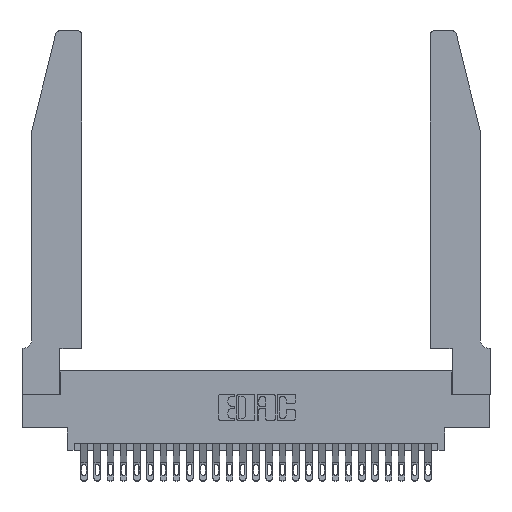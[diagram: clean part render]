
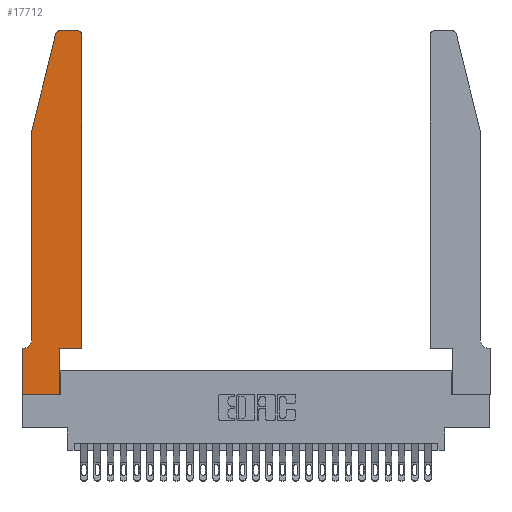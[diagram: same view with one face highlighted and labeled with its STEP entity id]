
A CAD part, top view. The second image highlights one B-rep face of the part: STEP entity #17712.
In plain terms, the highlighted planar face has unit normal (0, 0, 1).
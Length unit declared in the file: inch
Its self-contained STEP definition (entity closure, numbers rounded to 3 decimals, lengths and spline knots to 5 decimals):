
#638 = DIRECTION ( 'NONE',  ( 1., 0., 0. ) ) ;
#938 = VERTEX_POINT ( 'NONE', #22571 ) ;
#1286 = VERTEX_POINT ( 'NONE', #9032 ) ;
#1405 = AXIS2_PLACEMENT_3D ( 'NONE', #23999, #10902, #26207 ) ;
#1491 = CARTESIAN_POINT ( 'NONE',  ( 0.2865, 0.35, 0.37 ) ) ;
#2032 = DIRECTION ( 'NONE',  ( 1., 0., 0. ) ) ;
#2390 = CARTESIAN_POINT ( 'NONE',  ( 0., 0., 0.37 ) ) ;
#2399 = VERTEX_POINT ( 'NONE', #20181 ) ;
#2743 = ORIENTED_EDGE ( 'NONE', *, *, #19692, .T. ) ;
#2772 = VERTEX_POINT ( 'NONE', #26494 ) ;
#2855 = CARTESIAN_POINT ( 'NONE',  ( 0.4505, 0.35, 0.37 ) ) ;
#3191 = VECTOR ( 'NONE', #9762, 39.37008 ) ;
#3210 = ORIENTED_EDGE ( 'NONE', *, *, #19323, .T. ) ;
#3526 = LINE ( 'NONE', #24696, #26150 ) ;
#4059 = ORIENTED_EDGE ( 'NONE', *, *, #17505, .T. ) ;
#4582 = CARTESIAN_POINT ( 'NONE',  ( 0.0755, 2., 0.37 ) ) ;
#4821 = LINE ( 'NONE', #14977, #21586 ) ;
#5049 = ORIENTED_EDGE ( 'NONE', *, *, #12039, .T. ) ;
#5088 = DIRECTION ( 'NONE',  ( 0., 1., 0. ) ) ;
#5116 = ORIENTED_EDGE ( 'NONE', *, *, #13300, .T. ) ;
#5153 = AXIS2_PLACEMENT_3D ( 'NONE', #17276, #15197, #2032 ) ;
#6018 = VECTOR ( 'NONE', #24577, 39.37008 ) ;
#6329 = EDGE_CURVE ( 'NONE', #21389, #938, #27459, .T. ) ;
#6726 = DIRECTION ( 'NONE',  ( -1., 0., 0. ) ) ;
#6856 = DIRECTION ( 'NONE',  ( 0., -1., 0. ) ) ;
#6885 = DIRECTION ( 'NONE',  ( 0., 0., -1. ) ) ;
#6930 = LINE ( 'NONE', #2390, #23001 ) ;
#7084 = CARTESIAN_POINT ( 'NONE',  ( 0.4505, 0.35, 0.37 ) ) ;
#7373 = CARTESIAN_POINT ( 'NONE',  ( 0.4205, 2.75, 0.37 ) ) ;
#7693 = VECTOR ( 'NONE', #6726, 39.37008 ) ;
#8584 = CIRCLE ( 'NONE', #25892, 0.07 ) ;
#9032 = CARTESIAN_POINT ( 'NONE',  ( 0.0055, 0.35, 0.37 ) ) ;
#9314 = VECTOR ( 'NONE', #5088, 39.37008 ) ;
#9665 = ORIENTED_EDGE ( 'NONE', *, *, #13156, .T. ) ;
#9762 = DIRECTION ( 'NONE',  ( 1., 0., 0. ) ) ;
#10742 = FACE_OUTER_BOUND ( 'NONE', #16281, .T. ) ;
#10902 = DIRECTION ( 'NONE',  ( 0., 0., 1. ) ) ;
#11002 = VECTOR ( 'NONE', #25261, 39.37008 ) ;
#11259 = ORIENTED_EDGE ( 'NONE', *, *, #19066, .T. ) ;
#11550 = VERTEX_POINT ( 'NONE', #18581 ) ;
#11599 = ORIENTED_EDGE ( 'NONE', *, *, #16405, .T. ) ;
#11856 = LINE ( 'NONE', #7084, #6018 ) ;
#12039 = EDGE_CURVE ( 'NONE', #28290, #21389, #11856, .T. ) ;
#12504 = AXIS2_PLACEMENT_3D ( 'NONE', #26952, #13868, #638 ) ;
#13156 = EDGE_CURVE ( 'NONE', #16662, #2772, #19318, .T. ) ;
#13300 = EDGE_CURVE ( 'NONE', #11550, #22076, #3526, .T. ) ;
#13771 = LINE ( 'NONE', #23049, #11002 ) ;
#13868 = DIRECTION ( 'NONE',  ( 0., 0., 1. ) ) ;
#14195 = CIRCLE ( 'NONE', #12504, 0.03 ) ;
#14228 = LINE ( 'NONE', #18942, #3191 ) ;
#14344 = ORIENTED_EDGE ( 'NONE', *, *, #18013, .T. ) ;
#14977 = CARTESIAN_POINT ( 'NONE',  ( 0.0755, 0.35, 0.37 ) ) ;
#15197 = DIRECTION ( 'NONE',  ( 0., 0., 1. ) ) ;
#15374 = EDGE_CURVE ( 'NONE', #19605, #24996, #6930, .T. ) ;
#15944 = CARTESIAN_POINT ( 'NONE',  ( 0.0755, 0.42, 0.37 ) ) ;
#16281 = EDGE_LOOP ( 'NONE', ( #9665, #14344, #5116, #11259, #2743, #23636, #17816, #4059, #3210, #5049, #23106, #11599 ) ) ;
#16405 = EDGE_CURVE ( 'NONE', #938, #16662, #24469, .T. ) ;
#16662 = VERTEX_POINT ( 'NONE', #7373 ) ;
#17276 = CARTESIAN_POINT ( 'NONE',  ( 0., 0.35, 0.37 ) ) ;
#17376 = CARTESIAN_POINT ( 'NONE',  ( 0., 0.35, 0.37 ) ) ;
#17505 = EDGE_CURVE ( 'NONE', #24996, #2399, #14228, .T. ) ;
#17712 = ADVANCED_FACE ( 'NONE', ( #10742 ), #28287, .T. ) ;
#17816 = ORIENTED_EDGE ( 'NONE', *, *, #15374, .T. ) ;
#17996 = VERTEX_POINT ( 'NONE', #15944 ) ;
#18013 = EDGE_CURVE ( 'NONE', #2772, #11550, #14195, .T. ) ;
#18558 = VECTOR ( 'NONE', #22092, 39.37008 ) ;
#18581 = CARTESIAN_POINT ( 'NONE',  ( 0.25487, 2.72718, 0.37 ) ) ;
#18942 = CARTESIAN_POINT ( 'NONE',  ( 0., 0., 0.37 ) ) ;
#19066 = EDGE_CURVE ( 'NONE', #22076, #17996, #24360, .T. ) ;
#19318 = LINE ( 'NONE', #21998, #7693 ) ;
#19323 = EDGE_CURVE ( 'NONE', #2399, #28290, #13771, .T. ) ;
#19605 = VERTEX_POINT ( 'NONE', #17376 ) ;
#19692 = EDGE_CURVE ( 'NONE', #17996, #1286, #8584, .T. ) ;
#19978 = CARTESIAN_POINT ( 'NONE',  ( 0.0055, 0.42, 0.37 ) ) ;
#20181 = CARTESIAN_POINT ( 'NONE',  ( 0.2865, 0., 0.37 ) ) ;
#21389 = VERTEX_POINT ( 'NONE', #27549 ) ;
#21586 = VECTOR ( 'NONE', #23666, 39.37008 ) ;
#21998 = CARTESIAN_POINT ( 'NONE',  ( 0.2605, 2.75, 0.37 ) ) ;
#22076 = VERTEX_POINT ( 'NONE', #27878 ) ;
#22092 = DIRECTION ( 'NONE',  ( 0., -1., 0. ) ) ;
#22157 = DIRECTION ( 'NONE',  ( -1., 0., 0. ) ) ;
#22571 = CARTESIAN_POINT ( 'NONE',  ( 0.4505, 2.72, 0.37 ) ) ;
#23001 = VECTOR ( 'NONE', #6856, 39.37008 ) ;
#23049 = CARTESIAN_POINT ( 'NONE',  ( 0.2865, 0.35, 0.37 ) ) ;
#23106 = ORIENTED_EDGE ( 'NONE', *, *, #6329, .T. ) ;
#23636 = ORIENTED_EDGE ( 'NONE', *, *, #23710, .T. ) ;
#23666 = DIRECTION ( 'NONE',  ( -1., 0., 0. ) ) ;
#23710 = EDGE_CURVE ( 'NONE', #1286, #19605, #4821, .T. ) ;
#23999 = CARTESIAN_POINT ( 'NONE',  ( 0.4205, 2.72, 0.37 ) ) ;
#24360 = LINE ( 'NONE', #4582, #18558 ) ;
#24469 = CIRCLE ( 'NONE', #1405, 0.03 ) ;
#24577 = DIRECTION ( 'NONE',  ( 1., 0., 0. ) ) ;
#24606 = DIRECTION ( 'NONE',  ( -0.239, -0.971, 0. ) ) ;
#24696 = CARTESIAN_POINT ( 'NONE',  ( 0.0755, 2., 0.37 ) ) ;
#24996 = VERTEX_POINT ( 'NONE', #25984 ) ;
#25261 = DIRECTION ( 'NONE',  ( 0., 1., 0. ) ) ;
#25892 = AXIS2_PLACEMENT_3D ( 'NONE', #19978, #6885, #22157 ) ;
#25984 = CARTESIAN_POINT ( 'NONE',  ( 0., 0., 0.37 ) ) ;
#26150 = VECTOR ( 'NONE', #24606, 39.37008 ) ;
#26207 = DIRECTION ( 'NONE',  ( 1., 0., 0. ) ) ;
#26494 = CARTESIAN_POINT ( 'NONE',  ( 0.284, 2.75, 0.37 ) ) ;
#26952 = CARTESIAN_POINT ( 'NONE',  ( 0.284, 2.72, 0.37 ) ) ;
#27459 = LINE ( 'NONE', #2855, #9314 ) ;
#27549 = CARTESIAN_POINT ( 'NONE',  ( 0.4505, 0.35, 0.37 ) ) ;
#27878 = CARTESIAN_POINT ( 'NONE',  ( 0.0755, 2., 0.37 ) ) ;
#28287 = PLANE ( 'NONE',  #5153 ) ;
#28290 = VERTEX_POINT ( 'NONE', #1491 ) ;
